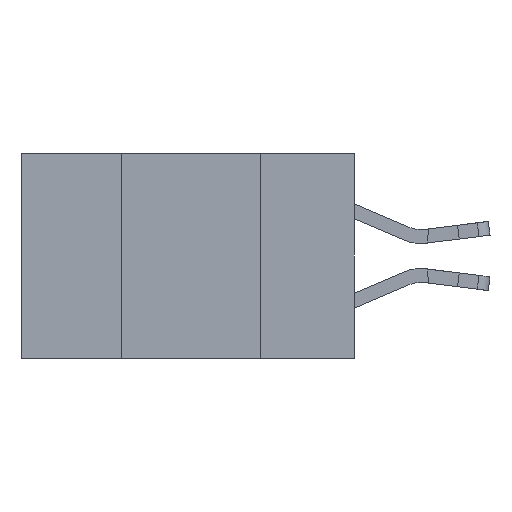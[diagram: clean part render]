
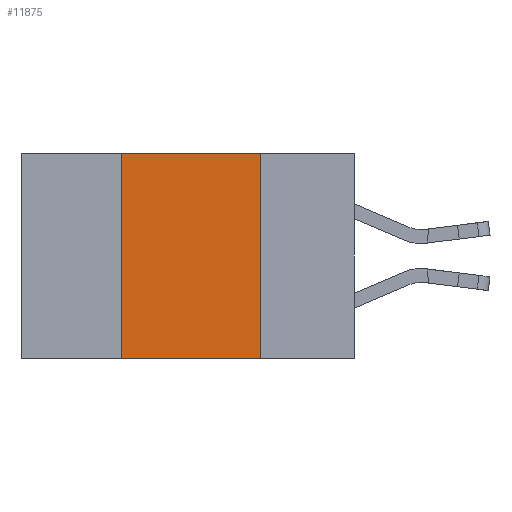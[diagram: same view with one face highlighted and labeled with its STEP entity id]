
A CAD part, left-side view. The second image highlights one B-rep face of the part: STEP entity #11875.
In plain terms, the highlighted planar face has unit normal (-1, 0, 0).
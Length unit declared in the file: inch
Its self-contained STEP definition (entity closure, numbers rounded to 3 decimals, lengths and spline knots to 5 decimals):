
#43 = VECTOR ( 'NONE', #5318, 39.37008 ) ;
#146 = LINE ( 'NONE', #8981, #7903 ) ;
#156 = VERTEX_POINT ( 'NONE', #230 ) ;
#230 = CARTESIAN_POINT ( 'NONE',  ( 0., 0.17, -0.37 ) ) ;
#739 = LINE ( 'NONE', #8481, #5414 ) ;
#1066 = CARTESIAN_POINT ( 'NONE',  ( 0., 0.6, 0. ) ) ;
#1136 = DIRECTION ( 'NONE',  ( 0., 0., -1. ) ) ;
#2066 = PLANE ( 'NONE',  #13039 ) ;
#3451 = DIRECTION ( 'NONE',  ( 0., -1., 0. ) ) ;
#3522 = CARTESIAN_POINT ( 'NONE',  ( 0., 0.17, 0. ) ) ;
#3672 = VERTEX_POINT ( 'NONE', #5433 ) ;
#3833 = EDGE_CURVE ( 'NONE', #5964, #156, #4783, .T. ) ;
#3926 = ORIENTED_EDGE ( 'NONE', *, *, #3833, .F. ) ;
#4783 = LINE ( 'NONE', #13627, #13597 ) ;
#5318 = DIRECTION ( 'NONE',  ( 0., -1., 0. ) ) ;
#5414 = VECTOR ( 'NONE', #8343, 39.37008 ) ;
#5433 = CARTESIAN_POINT ( 'NONE',  ( 0., 0.42, -0.37 ) ) ;
#5456 = DIRECTION ( 'NONE',  ( 1., 0., 0. ) ) ;
#5964 = VERTEX_POINT ( 'NONE', #3522 ) ;
#6821 = DIRECTION ( 'NONE',  ( 0., 0., -1. ) ) ;
#7903 = VECTOR ( 'NONE', #3451, 39.37008 ) ;
#8081 = EDGE_LOOP ( 'NONE', ( #3926, #11505, #13845, #10994 ) ) ;
#8343 = DIRECTION ( 'NONE',  ( 0., 0., 1. ) ) ;
#8458 = LINE ( 'NONE', #8529, #43 ) ;
#8481 = CARTESIAN_POINT ( 'NONE',  ( 0., 0.42, -0.37 ) ) ;
#8529 = CARTESIAN_POINT ( 'NONE',  ( 0., 0.6, 0. ) ) ;
#8674 = EDGE_CURVE ( 'NONE', #3672, #156, #146, .T. ) ;
#8981 = CARTESIAN_POINT ( 'NONE',  ( 0., 0.6, -0.37 ) ) ;
#9001 = VERTEX_POINT ( 'NONE', #10620 ) ;
#10131 = EDGE_CURVE ( 'NONE', #9001, #5964, #8458, .T. ) ;
#10620 = CARTESIAN_POINT ( 'NONE',  ( 0., 0.42, 0. ) ) ;
#10994 = ORIENTED_EDGE ( 'NONE', *, *, #8674, .T. ) ;
#11505 = ORIENTED_EDGE ( 'NONE', *, *, #10131, .F. ) ;
#11875 = ADVANCED_FACE ( 'NONE', ( #11996 ), #2066, .F. ) ;
#11996 = FACE_OUTER_BOUND ( 'NONE', #8081, .T. ) ;
#13039 = AXIS2_PLACEMENT_3D ( 'NONE', #1066, #5456, #1136 ) ;
#13597 = VECTOR ( 'NONE', #6821, 39.37008 ) ;
#13627 = CARTESIAN_POINT ( 'NONE',  ( 0., 0.17, -0.37 ) ) ;
#13845 = ORIENTED_EDGE ( 'NONE', *, *, #13874, .F. ) ;
#13874 = EDGE_CURVE ( 'NONE', #3672, #9001, #739, .T. ) ;
